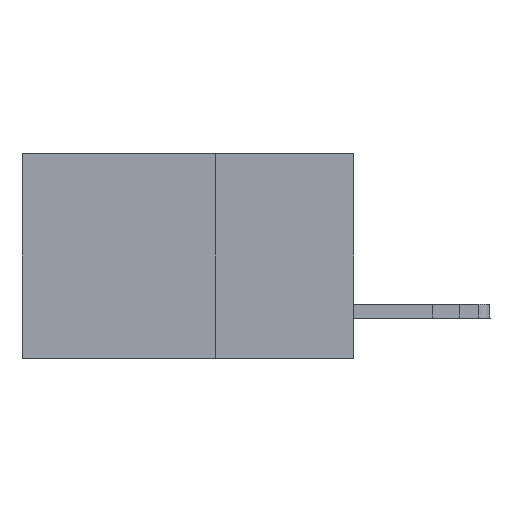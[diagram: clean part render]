
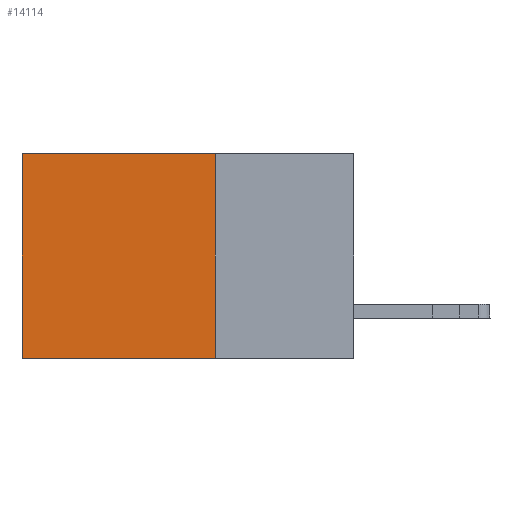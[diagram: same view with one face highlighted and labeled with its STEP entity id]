
A CAD part, left-side view. The second image highlights one B-rep face of the part: STEP entity #14114.
In plain terms, the highlighted planar face has unit normal (-1, 0, 0).
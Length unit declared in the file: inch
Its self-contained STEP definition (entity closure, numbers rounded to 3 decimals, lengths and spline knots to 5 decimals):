
#848 = LINE ( 'NONE', #1015, #26354 ) ;
#1015 = CARTESIAN_POINT ( 'NONE',  ( 0.2875, 0.6, 0. ) ) ;
#3011 = DIRECTION ( 'NONE',  ( 1., 0., 0. ) ) ;
#3176 = FACE_OUTER_BOUND ( 'NONE', #13888, .T. ) ;
#4485 = VECTOR ( 'NONE', #7264, 39.37008 ) ;
#6374 = VERTEX_POINT ( 'NONE', #14363 ) ;
#7110 = CARTESIAN_POINT ( 'NONE',  ( 0.2875, 0.25, -0.37 ) ) ;
#7264 = DIRECTION ( 'NONE',  ( 0., 1., 0. ) ) ;
#8504 = DIRECTION ( 'NONE',  ( 0., 0., -1. ) ) ;
#9286 = CARTESIAN_POINT ( 'NONE',  ( 0.2875, 0.25, 0. ) ) ;
#10220 = AXIS2_PLACEMENT_3D ( 'NONE', #29635, #3011, #22314 ) ;
#10869 = ORIENTED_EDGE ( 'NONE', *, *, #11017, .T. ) ;
#11017 = EDGE_CURVE ( 'NONE', #21628, #14815, #848, .T. ) ;
#12355 = ORIENTED_EDGE ( 'NONE', *, *, #30045, .F. ) ;
#12430 = PLANE ( 'NONE',  #10220 ) ;
#12532 = ORIENTED_EDGE ( 'NONE', *, *, #24593, .F. ) ;
#12897 = VERTEX_POINT ( 'NONE', #30628 ) ;
#13888 = EDGE_LOOP ( 'NONE', ( #10869, #12532, #12355, #30827 ) ) ;
#14114 = ADVANCED_FACE ( 'NONE', ( #3176 ), #12430, .F. ) ;
#14363 = CARTESIAN_POINT ( 'NONE',  ( 0.2875, 0.25, -0.37 ) ) ;
#14815 = VERTEX_POINT ( 'NONE', #22273 ) ;
#15386 = VECTOR ( 'NONE', #26653, 39.37008 ) ;
#15885 = VECTOR ( 'NONE', #24721, 39.37008 ) ;
#17559 = CARTESIAN_POINT ( 'NONE',  ( 0.2875, 0.25, 0. ) ) ;
#19408 = LINE ( 'NONE', #7110, #4485 ) ;
#21411 = LINE ( 'NONE', #9286, #15386 ) ;
#21628 = VERTEX_POINT ( 'NONE', #23758 ) ;
#22179 = LINE ( 'NONE', #17559, #15885 ) ;
#22273 = CARTESIAN_POINT ( 'NONE',  ( 0.2875, 0.6, -0.37 ) ) ;
#22314 = DIRECTION ( 'NONE',  ( 0., 0., -1. ) ) ;
#23758 = CARTESIAN_POINT ( 'NONE',  ( 0.2875, 0.6, 0. ) ) ;
#24593 = EDGE_CURVE ( 'NONE', #6374, #14815, #19408, .T. ) ;
#24721 = DIRECTION ( 'NONE',  ( 0., 1., 0. ) ) ;
#26354 = VECTOR ( 'NONE', #8504, 39.37008 ) ;
#26653 = DIRECTION ( 'NONE',  ( 0., 0., -1. ) ) ;
#28260 = EDGE_CURVE ( 'NONE', #12897, #21628, #22179, .T. ) ;
#29635 = CARTESIAN_POINT ( 'NONE',  ( 0.2875, 0.25, 0. ) ) ;
#30045 = EDGE_CURVE ( 'NONE', #12897, #6374, #21411, .T. ) ;
#30628 = CARTESIAN_POINT ( 'NONE',  ( 0.2875, 0.25, 0. ) ) ;
#30827 = ORIENTED_EDGE ( 'NONE', *, *, #28260, .T. ) ;
